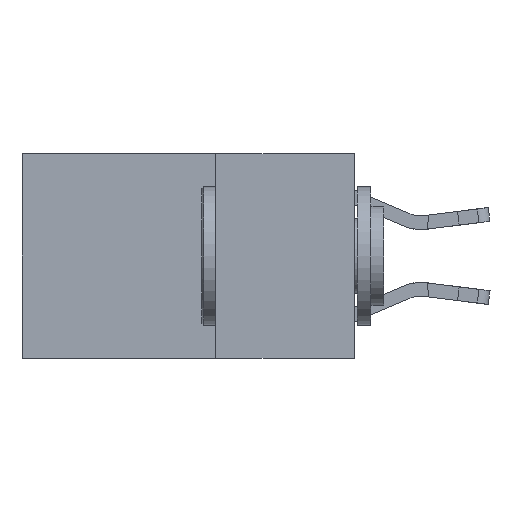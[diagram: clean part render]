
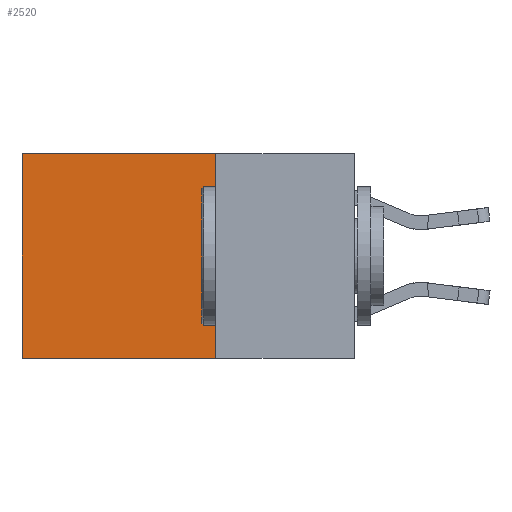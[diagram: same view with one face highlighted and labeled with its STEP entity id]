
A CAD part, left-side view. The second image highlights one B-rep face of the part: STEP entity #2520.
In plain terms, the highlighted planar face has unit normal (-1, 0, 0).
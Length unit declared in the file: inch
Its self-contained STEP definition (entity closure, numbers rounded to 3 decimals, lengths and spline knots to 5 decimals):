
#2520 = ADVANCED_FACE ( 'NONE', ( #17914 ), #6488, .F. ) ;
#2638 = ORIENTED_EDGE ( 'NONE', *, *, #20080, .T. ) ;
#3027 = VECTOR ( 'NONE', #11861, 39.37008 ) ;
#3166 = CARTESIAN_POINT ( 'NONE',  ( 0.2625, 0.6, -0.37 ) ) ;
#4471 = EDGE_CURVE ( 'NONE', #8250, #12613, #7689, .T. ) ;
#4474 = EDGE_LOOP ( 'NONE', ( #2638, #10939, #18534, #16773 ) ) ;
#5591 = CARTESIAN_POINT ( 'NONE',  ( 0.2625, 0.25, 0. ) ) ;
#6333 = DIRECTION ( 'NONE',  ( 0., 0., -1. ) ) ;
#6334 = DIRECTION ( 'NONE',  ( 1., 0., 0. ) ) ;
#6402 = VERTEX_POINT ( 'NONE', #12813 ) ;
#6488 = PLANE ( 'NONE',  #7581 ) ;
#6645 = CARTESIAN_POINT ( 'NONE',  ( 0.2625, 0.25, 0. ) ) ;
#6653 = VECTOR ( 'NONE', #9432, 39.37008 ) ;
#7581 = AXIS2_PLACEMENT_3D ( 'NONE', #6645, #6334, #6333 ) ;
#7689 = LINE ( 'NONE', #5591, #3027 ) ;
#8211 = VECTOR ( 'NONE', #20092, 39.37008 ) ;
#8250 = VERTEX_POINT ( 'NONE', #15600 ) ;
#9003 = LINE ( 'NONE', #9262, #12615 ) ;
#9262 = CARTESIAN_POINT ( 'NONE',  ( 0.2625, 0.25, -0.37 ) ) ;
#9405 = EDGE_CURVE ( 'NONE', #6402, #17760, #9003, .T. ) ;
#9432 = DIRECTION ( 'NONE',  ( 0., 0., -1. ) ) ;
#10105 = EDGE_CURVE ( 'NONE', #8250, #6402, #12363, .T. ) ;
#10939 = ORIENTED_EDGE ( 'NONE', *, *, #9405, .F. ) ;
#11861 = DIRECTION ( 'NONE',  ( 0., 1., 0. ) ) ;
#12363 = LINE ( 'NONE', #15454, #8211 ) ;
#12371 = DIRECTION ( 'NONE',  ( 0., 1., 0. ) ) ;
#12613 = VERTEX_POINT ( 'NONE', #12784 ) ;
#12615 = VECTOR ( 'NONE', #12371, 39.37008 ) ;
#12784 = CARTESIAN_POINT ( 'NONE',  ( 0.2625, 0.6, 0. ) ) ;
#12813 = CARTESIAN_POINT ( 'NONE',  ( 0.2625, 0.25, -0.37 ) ) ;
#13963 = CARTESIAN_POINT ( 'NONE',  ( 0.2625, 0.6, 0. ) ) ;
#15454 = CARTESIAN_POINT ( 'NONE',  ( 0.2625, 0.25, 0. ) ) ;
#15600 = CARTESIAN_POINT ( 'NONE',  ( 0.2625, 0.25, 0. ) ) ;
#16773 = ORIENTED_EDGE ( 'NONE', *, *, #4471, .T. ) ;
#17760 = VERTEX_POINT ( 'NONE', #3166 ) ;
#17914 = FACE_OUTER_BOUND ( 'NONE', #4474, .T. ) ;
#18534 = ORIENTED_EDGE ( 'NONE', *, *, #10105, .F. ) ;
#19918 = LINE ( 'NONE', #13963, #6653 ) ;
#20080 = EDGE_CURVE ( 'NONE', #12613, #17760, #19918, .T. ) ;
#20092 = DIRECTION ( 'NONE',  ( 0., 0., -1. ) ) ;
